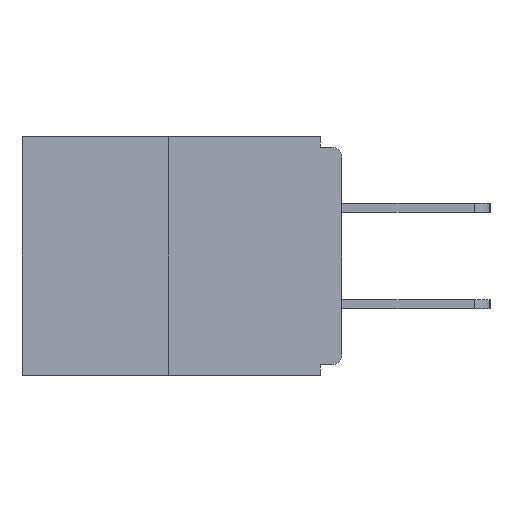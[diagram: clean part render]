
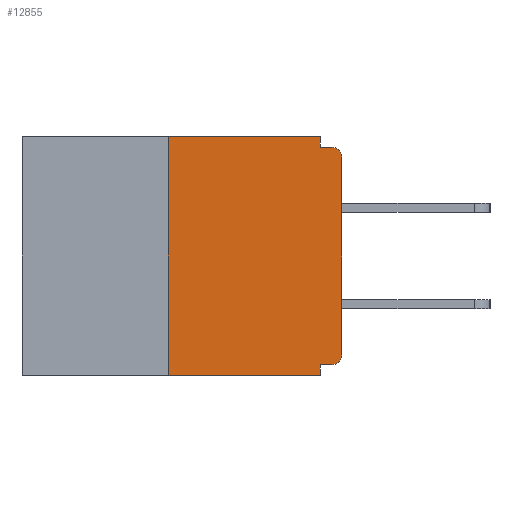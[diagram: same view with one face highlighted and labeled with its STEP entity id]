
A CAD part, left-side view. The second image highlights one B-rep face of the part: STEP entity #12855.
In plain terms, the highlighted planar face has unit normal (-1, 0, 0).
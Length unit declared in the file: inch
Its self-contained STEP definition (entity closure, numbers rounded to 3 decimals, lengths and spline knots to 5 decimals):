
#188 = LINE ( 'NONE', #18688, #17499 ) ;
#199 = CIRCLE ( 'NONE', #6257, 0.015 ) ;
#587 = VERTEX_POINT ( 'NONE', #3416 ) ;
#625 = EDGE_CURVE ( 'NONE', #24648, #7371, #17647, .T. ) ;
#937 = CIRCLE ( 'NONE', #14349, 0.015 ) ;
#1479 = VECTOR ( 'NONE', #23004, 39.37008 ) ;
#1672 = CARTESIAN_POINT ( 'NONE',  ( 0., 0.031, -0.343 ) ) ;
#1713 = VECTOR ( 'NONE', #24559, 39.37008 ) ;
#1741 = ORIENTED_EDGE ( 'NONE', *, *, #1827, .F. ) ;
#1827 = EDGE_CURVE ( 'NONE', #28966, #30235, #10398, .T. ) ;
#1915 = CARTESIAN_POINT ( 'NONE',  ( 0., 0.015, -0.03 ) ) ;
#2177 = ORIENTED_EDGE ( 'NONE', *, *, #27461, .T. ) ;
#2257 = CARTESIAN_POINT ( 'NONE',  ( 0., 0., -0.03 ) ) ;
#2570 = CARTESIAN_POINT ( 'NONE',  ( 0., 0.015, -0.015 ) ) ;
#2761 = CARTESIAN_POINT ( 'NONE',  ( 0., 0.031, 0. ) ) ;
#2967 = LINE ( 'NONE', #22798, #1479 ) ;
#3416 = CARTESIAN_POINT ( 'NONE',  ( 0., 0.25, 0. ) ) ;
#3527 = DIRECTION ( 'NONE',  ( 0., -1., 0. ) ) ;
#3632 = CARTESIAN_POINT ( 'NONE',  ( 0., 0., -0.328 ) ) ;
#4189 = EDGE_CURVE ( 'NONE', #7988, #587, #17851, .T. ) ;
#4267 = ORIENTED_EDGE ( 'NONE', *, *, #625, .F. ) ;
#4416 = CARTESIAN_POINT ( 'NONE',  ( 0., 0.46, 0. ) ) ;
#4440 = DIRECTION ( 'NONE',  ( 0., 0., -1. ) ) ;
#4811 = EDGE_CURVE ( 'NONE', #587, #21834, #188, .T. ) ;
#5221 = VECTOR ( 'NONE', #3527, 39.37008 ) ;
#5308 = CARTESIAN_POINT ( 'NONE',  ( 0., 0.031, -0.343 ) ) ;
#5334 = EDGE_LOOP ( 'NONE', ( #27057, #18896, #6250, #5473, #1741, #2177, #13889, #14946, #4267, #7658 ) ) ;
#5473 = ORIENTED_EDGE ( 'NONE', *, *, #20281, .F. ) ;
#6250 = ORIENTED_EDGE ( 'NONE', *, *, #13030, .T. ) ;
#6257 = AXIS2_PLACEMENT_3D ( 'NONE', #1915, #21178, #4440 ) ;
#6943 = AXIS2_PLACEMENT_3D ( 'NONE', #4416, #11545, #13869 ) ;
#7324 = VERTEX_POINT ( 'NONE', #2257 ) ;
#7371 = VERTEX_POINT ( 'NONE', #2570 ) ;
#7467 = FACE_OUTER_BOUND ( 'NONE', #5334, .T. ) ;
#7658 = ORIENTED_EDGE ( 'NONE', *, *, #9632, .F. ) ;
#7988 = VERTEX_POINT ( 'NONE', #13366 ) ;
#8232 = CARTESIAN_POINT ( 'NONE',  ( 0., 0., -0.015 ) ) ;
#8643 = VERTEX_POINT ( 'NONE', #10463 ) ;
#9632 = EDGE_CURVE ( 'NONE', #21834, #24648, #28450, .T. ) ;
#9642 = CARTESIAN_POINT ( 'NONE',  ( 0., 0., 0. ) ) ;
#10398 = LINE ( 'NONE', #3632, #27388 ) ;
#10463 = CARTESIAN_POINT ( 'NONE',  ( 0., 0., -0.313 ) ) ;
#11423 = VERTEX_POINT ( 'NONE', #1672 ) ;
#11545 = DIRECTION ( 'NONE',  ( 1., 0., 0. ) ) ;
#12831 = CARTESIAN_POINT ( 'NONE',  ( 0., 0.031, -0.328 ) ) ;
#12855 = ADVANCED_FACE ( 'NONE', ( #7467 ), #25899, .F. ) ;
#13030 = EDGE_CURVE ( 'NONE', #7988, #11423, #2967, .T. ) ;
#13366 = CARTESIAN_POINT ( 'NONE',  ( 0., 0.25, -0.343 ) ) ;
#13869 = DIRECTION ( 'NONE',  ( 0., 0., -1. ) ) ;
#13889 = ORIENTED_EDGE ( 'NONE', *, *, #25987, .T. ) ;
#14134 = DIRECTION ( 'NONE',  ( 0., -1., 0. ) ) ;
#14349 = AXIS2_PLACEMENT_3D ( 'NONE', #17870, #20617, #20291 ) ;
#14946 = ORIENTED_EDGE ( 'NONE', *, *, #27322, .T. ) ;
#17499 = VECTOR ( 'NONE', #14134, 39.37008 ) ;
#17647 = LINE ( 'NONE', #8232, #5221 ) ;
#17705 = VECTOR ( 'NONE', #29530, 39.37008 ) ;
#17851 = LINE ( 'NONE', #19496, #25796 ) ;
#17870 = CARTESIAN_POINT ( 'NONE',  ( 0., 0.015, -0.313 ) ) ;
#18624 = VECTOR ( 'NONE', #28929, 39.37008 ) ;
#18688 = CARTESIAN_POINT ( 'NONE',  ( 0., 0.46, 0. ) ) ;
#18896 = ORIENTED_EDGE ( 'NONE', *, *, #4189, .F. ) ;
#19496 = CARTESIAN_POINT ( 'NONE',  ( 0., 0.25, 0. ) ) ;
#20281 = EDGE_CURVE ( 'NONE', #30235, #11423, #29017, .T. ) ;
#20291 = DIRECTION ( 'NONE',  ( 0., 0., -1. ) ) ;
#20617 = DIRECTION ( 'NONE',  ( -1., 0., 0. ) ) ;
#21178 = DIRECTION ( 'NONE',  ( -1., 0., 0. ) ) ;
#21834 = VERTEX_POINT ( 'NONE', #25876 ) ;
#22729 = LINE ( 'NONE', #9642, #18624 ) ;
#22798 = CARTESIAN_POINT ( 'NONE',  ( 0., 0.46, -0.343 ) ) ;
#23004 = DIRECTION ( 'NONE',  ( 0., -1., 0. ) ) ;
#23348 = CARTESIAN_POINT ( 'NONE',  ( 0., 0.031, -0.015 ) ) ;
#24235 = DIRECTION ( 'NONE',  ( 0., 0., 1. ) ) ;
#24559 = DIRECTION ( 'NONE',  ( 0., 0., -1. ) ) ;
#24648 = VERTEX_POINT ( 'NONE', #23348 ) ;
#25796 = VECTOR ( 'NONE', #24235, 39.37008 ) ;
#25876 = CARTESIAN_POINT ( 'NONE',  ( 0., 0.031, 0. ) ) ;
#25899 = PLANE ( 'NONE',  #6943 ) ;
#25987 = EDGE_CURVE ( 'NONE', #8643, #7324, #22729, .T. ) ;
#27057 = ORIENTED_EDGE ( 'NONE', *, *, #4811, .F. ) ;
#27059 = CARTESIAN_POINT ( 'NONE',  ( 0., 0.015, -0.328 ) ) ;
#27322 = EDGE_CURVE ( 'NONE', #7324, #7371, #199, .T. ) ;
#27388 = VECTOR ( 'NONE', #27823, 39.37008 ) ;
#27461 = EDGE_CURVE ( 'NONE', #28966, #8643, #937, .T. ) ;
#27823 = DIRECTION ( 'NONE',  ( 0., 1., 0. ) ) ;
#28450 = LINE ( 'NONE', #2761, #1713 ) ;
#28929 = DIRECTION ( 'NONE',  ( 0., 0., 1. ) ) ;
#28966 = VERTEX_POINT ( 'NONE', #27059 ) ;
#29017 = LINE ( 'NONE', #5308, #17705 ) ;
#29530 = DIRECTION ( 'NONE',  ( 0., 0., -1. ) ) ;
#30235 = VERTEX_POINT ( 'NONE', #12831 ) ;
